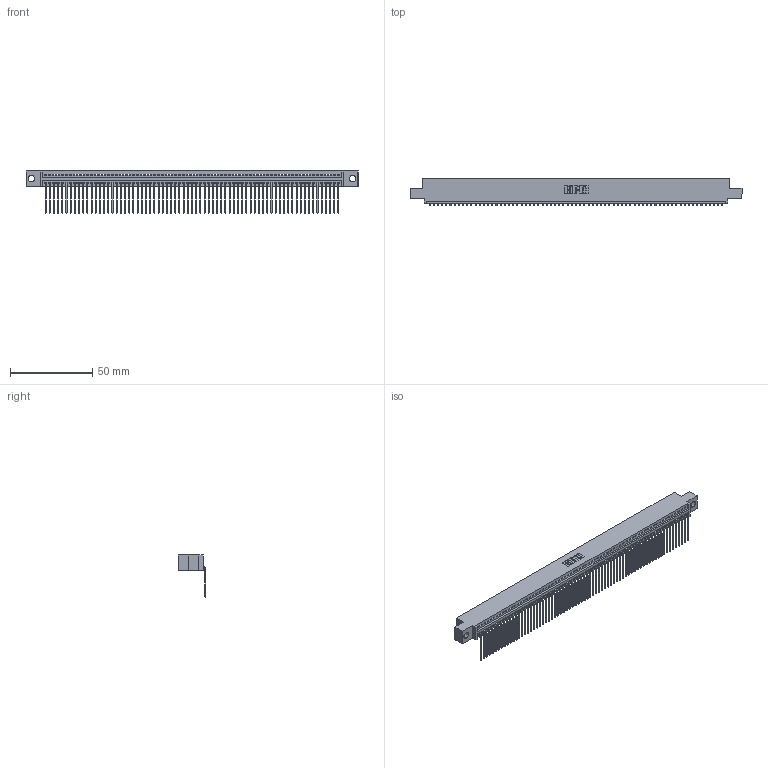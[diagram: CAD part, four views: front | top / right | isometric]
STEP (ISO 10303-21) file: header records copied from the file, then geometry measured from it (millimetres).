
FILE_DESCRIPTION (( 'STEP AP203' ), '1' );
FILE_NAME ('395-071-559-404.STEP', '2019-10-26T07:00:47', ( '' ), ( '' ), 'SwSTEP 2.0', 'SolidWorks 2016', '' );
FILE_SCHEMA (( 'CONFIG_CONTROL_DESIGN' ));
Length unit declared in the file: inch
Products named in the file (3): 395-071-559-404; 345 Part_0.110 Offset - 0.156 Dia-TH; 345-292-001_558 559 Tail - 1
Assembly tree (72 placements, depth 2):
  395-071-559-404
    345 Part_0.110 Offset - 0.156 Dia-TH
    345-292-001_558 559 Tail - 1  x71
Bounding box: 201.55 x 16.75 x 25.53 mm (x, y, z)
Volume: 19456.2 mm3; surface area: 27530.4 mm2
Topology: 72 solids, 72 shells, 4390 faces, 13275 edges, 8754 vertices
Faces by surface type: plane 3066, cylinder 1324
Entity records: 49751 total; most frequent: ORIENTED_EDGE 8630, CARTESIAN_POINT 8625, DIRECTION 7489, EDGE_CURVE 4315, VECTOR 3899, LINE 3899, VERTEX_POINT 2874, AXIS2_PLACEMENT_3D 1795
